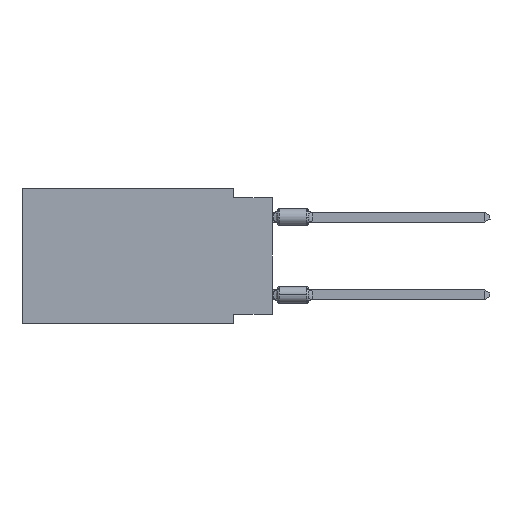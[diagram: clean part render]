
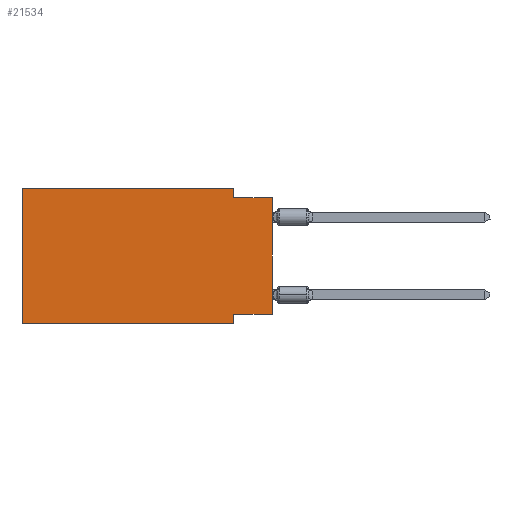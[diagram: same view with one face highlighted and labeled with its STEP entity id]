
A CAD part, left-side view. The second image highlights one B-rep face of the part: STEP entity #21534.
In plain terms, the highlighted planar face has unit normal (-1, 0, 0).
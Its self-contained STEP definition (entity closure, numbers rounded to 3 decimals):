
#1206 = EDGE_CURVE ( 'NONE', #34900, #39022, #73538, .T. ) ;
#1789 = CARTESIAN_POINT ( 'NONE',  ( 0., 16.383, 0. ) ) ;
#3674 = CARTESIAN_POINT ( 'NONE',  ( 0., 2.54, 0. ) ) ;
#4261 = VECTOR ( 'NONE', #48341, 1000. ) ;
#6919 = ORIENTED_EDGE ( 'NONE', *, *, #1206, .F. ) ;
#9096 = EDGE_CURVE ( 'NONE', #49211, #57542, #29010, .T. ) ;
#11592 = VECTOR ( 'NONE', #50831, 1000. ) ;
#12242 = DIRECTION ( 'NONE',  ( 0., 0., 1. ) ) ;
#12882 = DIRECTION ( 'NONE',  ( 0., 0., -1. ) ) ;
#12951 = FACE_OUTER_BOUND ( 'NONE', #50631, .T. ) ;
#13068 = VECTOR ( 'NONE', #34985, 1000. ) ;
#14046 = DIRECTION ( 'NONE',  ( 0., 0., -1. ) ) ;
#14894 = EDGE_CURVE ( 'NONE', #37209, #57542, #28646, .T. ) ;
#16324 = CARTESIAN_POINT ( 'NONE',  ( 0., 2.54, -0.635 ) ) ;
#17230 = LINE ( 'NONE', #57079, #58858 ) ;
#18897 = DIRECTION ( 'NONE',  ( 1., 0., 0. ) ) ;
#19113 = CARTESIAN_POINT ( 'NONE',  ( 0., 16.383, 0. ) ) ;
#21534 = ADVANCED_FACE ( 'NONE', ( #12951 ), #52065, .F. ) ;
#22288 = CARTESIAN_POINT ( 'NONE',  ( 0., 2.54, -8.89 ) ) ;
#23562 = DIRECTION ( 'NONE',  ( 0., -1., 0. ) ) ;
#24132 = CARTESIAN_POINT ( 'NONE',  ( 0., 16.383, 0. ) ) ;
#28122 = CARTESIAN_POINT ( 'NONE',  ( 0., 2.54, -8.89 ) ) ;
#28274 = CARTESIAN_POINT ( 'NONE',  ( 0., 0., 0. ) ) ;
#28646 = LINE ( 'NONE', #28274, #51689 ) ;
#29010 = LINE ( 'NONE', #68854, #13068 ) ;
#30100 = LINE ( 'NONE', #1789, #59093 ) ;
#31052 = EDGE_CURVE ( 'NONE', #68421, #40193, #17230, .T. ) ;
#31213 = LINE ( 'NONE', #53939, #4261 ) ;
#32348 = VERTEX_POINT ( 'NONE', #47512 ) ;
#33633 = VECTOR ( 'NONE', #42075, 1000. ) ;
#34900 = VERTEX_POINT ( 'NONE', #70434 ) ;
#34985 = DIRECTION ( 'NONE',  ( 0., -1., 0. ) ) ;
#35809 = ORIENTED_EDGE ( 'NONE', *, *, #9096, .F. ) ;
#36125 = LINE ( 'NONE', #58837, #33633 ) ;
#36792 = DIRECTION ( 'NONE',  ( 0., 0., 1. ) ) ;
#37209 = VERTEX_POINT ( 'NONE', #70095 ) ;
#39022 = VERTEX_POINT ( 'NONE', #22288 ) ;
#40193 = VERTEX_POINT ( 'NONE', #3674 ) ;
#41166 = ORIENTED_EDGE ( 'NONE', *, *, #63235, .F. ) ;
#41192 = LINE ( 'NONE', #63899, #50490 ) ;
#42075 = DIRECTION ( 'NONE',  ( 0., -1., 0. ) ) ;
#43716 = ORIENTED_EDGE ( 'NONE', *, *, #31052, .F. ) ;
#43928 = ORIENTED_EDGE ( 'NONE', *, *, #14894, .T. ) ;
#47512 = CARTESIAN_POINT ( 'NONE',  ( 0., 16.383, -8.89 ) ) ;
#48341 = DIRECTION ( 'NONE',  ( 0., 1., 0. ) ) ;
#49211 = VERTEX_POINT ( 'NONE', #16324 ) ;
#50490 = VECTOR ( 'NONE', #12882, 1000. ) ;
#50631 = EDGE_LOOP ( 'NONE', ( #43928, #35809, #51992, #43716, #41166, #65764, #6919, #57383 ) ) ;
#50831 = DIRECTION ( 'NONE',  ( 0., 0., -1. ) ) ;
#51689 = VECTOR ( 'NONE', #12242, 1000. ) ;
#51992 = ORIENTED_EDGE ( 'NONE', *, *, #66665, .F. ) ;
#52065 = PLANE ( 'NONE',  #54831 ) ;
#53939 = CARTESIAN_POINT ( 'NONE',  ( 0., 0., -8.255 ) ) ;
#54490 = EDGE_CURVE ( 'NONE', #37209, #34900, #31213, .T. ) ;
#54831 = AXIS2_PLACEMENT_3D ( 'NONE', #24132, #18897, #14046 ) ;
#57079 = CARTESIAN_POINT ( 'NONE',  ( 0., 16.383, 0. ) ) ;
#57383 = ORIENTED_EDGE ( 'NONE', *, *, #54490, .F. ) ;
#57542 = VERTEX_POINT ( 'NONE', #64206 ) ;
#58837 = CARTESIAN_POINT ( 'NONE',  ( 0., 16.383, -8.89 ) ) ;
#58858 = VECTOR ( 'NONE', #23562, 1000. ) ;
#59093 = VECTOR ( 'NONE', #36792, 1000. ) ;
#63235 = EDGE_CURVE ( 'NONE', #32348, #68421, #30100, .T. ) ;
#63899 = CARTESIAN_POINT ( 'NONE',  ( 0., 2.54, 0. ) ) ;
#64206 = CARTESIAN_POINT ( 'NONE',  ( 0., 0., -0.635 ) ) ;
#65764 = ORIENTED_EDGE ( 'NONE', *, *, #71517, .T. ) ;
#66665 = EDGE_CURVE ( 'NONE', #40193, #49211, #41192, .T. ) ;
#68421 = VERTEX_POINT ( 'NONE', #19113 ) ;
#68854 = CARTESIAN_POINT ( 'NONE',  ( 0., 0., -0.635 ) ) ;
#70095 = CARTESIAN_POINT ( 'NONE',  ( 0., 0., -8.255 ) ) ;
#70434 = CARTESIAN_POINT ( 'NONE',  ( 0., 2.54, -8.255 ) ) ;
#71517 = EDGE_CURVE ( 'NONE', #32348, #39022, #36125, .T. ) ;
#73538 = LINE ( 'NONE', #28122, #11592 ) ;
